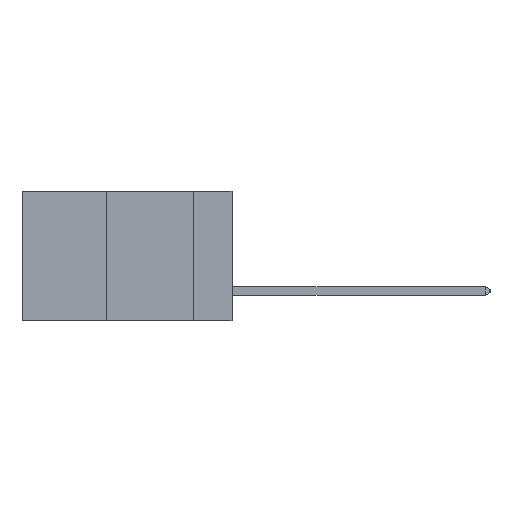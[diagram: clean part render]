
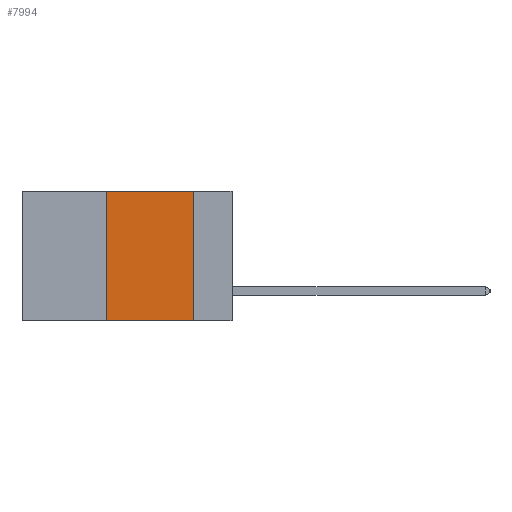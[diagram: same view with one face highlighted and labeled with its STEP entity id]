
A CAD part, left-side view. The second image highlights one B-rep face of the part: STEP entity #7994.
In plain terms, the highlighted planar face has unit normal (-1, 0, 0).
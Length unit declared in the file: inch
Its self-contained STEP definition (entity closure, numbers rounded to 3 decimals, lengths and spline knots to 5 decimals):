
#1638 = EDGE_CURVE ( 'NONE', #24655, #25323, #9463, .T. ) ;
#4601 = VECTOR ( 'NONE', #10798, 39.37008 ) ;
#7634 = CARTESIAN_POINT ( 'NONE',  ( 0., 0.6, 0. ) ) ;
#7994 = ADVANCED_FACE ( 'NONE', ( #22850 ), #19672, .F. ) ;
#9463 = LINE ( 'NONE', #25117, #4601 ) ;
#10798 = DIRECTION ( 'NONE',  ( 0., 0., -1. ) ) ;
#11152 = CARTESIAN_POINT ( 'NONE',  ( 0., 0.11, -0.37 ) ) ;
#11466 = DIRECTION ( 'NONE',  ( 1., 0., 0. ) ) ;
#11841 = CARTESIAN_POINT ( 'NONE',  ( 0., 0.36, -0.37 ) ) ;
#12293 = CARTESIAN_POINT ( 'NONE',  ( 0., 0.36, 0. ) ) ;
#13008 = EDGE_LOOP ( 'NONE', ( #16906, #16261, #20450, #13446 ) ) ;
#13318 = VECTOR ( 'NONE', #18576, 39.37008 ) ;
#13446 = ORIENTED_EDGE ( 'NONE', *, *, #18525, .T. ) ;
#14312 = LINE ( 'NONE', #12293, #24475 ) ;
#14469 = CARTESIAN_POINT ( 'NONE',  ( 0., 0.6, -0.37 ) ) ;
#14647 = LINE ( 'NONE', #14469, #13318 ) ;
#16261 = ORIENTED_EDGE ( 'NONE', *, *, #21785, .F. ) ;
#16906 = ORIENTED_EDGE ( 'NONE', *, *, #1638, .F. ) ;
#18525 = EDGE_CURVE ( 'NONE', #18993, #25323, #14647, .T. ) ;
#18576 = DIRECTION ( 'NONE',  ( 0., -1., 0. ) ) ;
#18888 = VECTOR ( 'NONE', #26246, 39.37008 ) ;
#18993 = VERTEX_POINT ( 'NONE', #11841 ) ;
#19672 = PLANE ( 'NONE',  #20542 ) ;
#20450 = ORIENTED_EDGE ( 'NONE', *, *, #23211, .F. ) ;
#20542 = AXIS2_PLACEMENT_3D ( 'NONE', #23755, #11466, #25785 ) ;
#20610 = VERTEX_POINT ( 'NONE', #25360 ) ;
#21785 = EDGE_CURVE ( 'NONE', #20610, #24655, #24244, .T. ) ;
#22850 = FACE_OUTER_BOUND ( 'NONE', #13008, .T. ) ;
#23134 = CARTESIAN_POINT ( 'NONE',  ( 0., 0.11, 0. ) ) ;
#23211 = EDGE_CURVE ( 'NONE', #18993, #20610, #14312, .T. ) ;
#23755 = CARTESIAN_POINT ( 'NONE',  ( 0., 0.6, 0. ) ) ;
#24244 = LINE ( 'NONE', #7634, #18888 ) ;
#24475 = VECTOR ( 'NONE', #26582, 39.37008 ) ;
#24655 = VERTEX_POINT ( 'NONE', #23134 ) ;
#25117 = CARTESIAN_POINT ( 'NONE',  ( 0., 0.11, 0. ) ) ;
#25323 = VERTEX_POINT ( 'NONE', #11152 ) ;
#25360 = CARTESIAN_POINT ( 'NONE',  ( 0., 0.36, 0. ) ) ;
#25785 = DIRECTION ( 'NONE',  ( 0., 0., -1. ) ) ;
#26246 = DIRECTION ( 'NONE',  ( 0., -1., 0. ) ) ;
#26582 = DIRECTION ( 'NONE',  ( 0., 0., 1. ) ) ;
